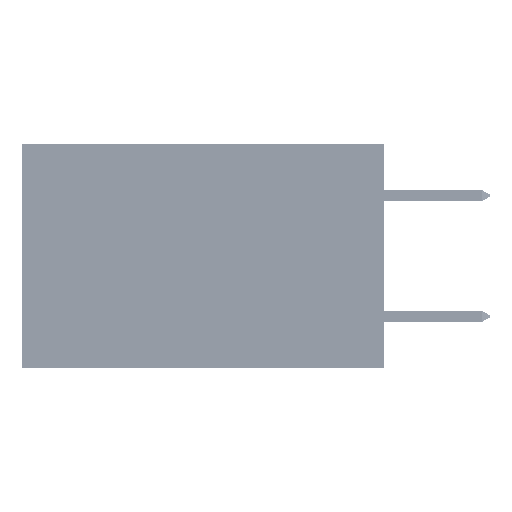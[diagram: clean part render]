
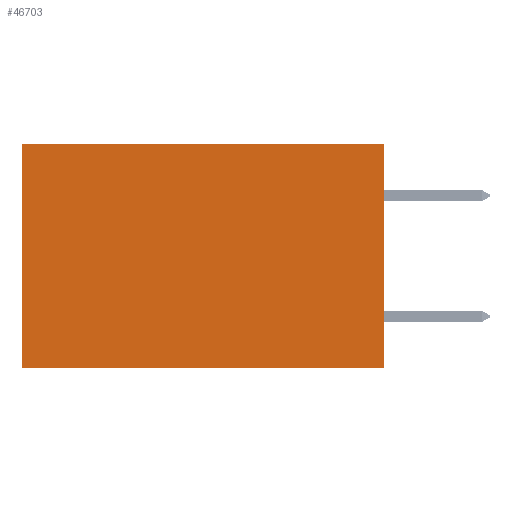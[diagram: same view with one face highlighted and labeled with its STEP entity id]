
A CAD part, left-side view. The second image highlights one B-rep face of the part: STEP entity #46703.
In plain terms, the highlighted planar face has unit normal (-1, 0, 0).
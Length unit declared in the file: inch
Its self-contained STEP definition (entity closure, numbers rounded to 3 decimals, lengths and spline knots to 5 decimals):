
#183 = CARTESIAN_POINT ( 'NONE',  ( 0.2875, 0., 0. ) ) ;
#894 = CARTESIAN_POINT ( 'NONE',  ( 0.2875, 0., -0.37 ) ) ;
#3247 = CARTESIAN_POINT ( 'NONE',  ( 0.2875, 0., 0. ) ) ;
#5212 = EDGE_LOOP ( 'NONE', ( #28532, #8149, #8912, #12407 ) ) ;
#7682 = PLANE ( 'NONE',  #45016 ) ;
#7982 = CARTESIAN_POINT ( 'NONE',  ( 0.2875, 0.6, 0. ) ) ;
#8149 = ORIENTED_EDGE ( 'NONE', *, *, #19596, .F. ) ;
#8912 = ORIENTED_EDGE ( 'NONE', *, *, #36815, .F. ) ;
#11177 = DIRECTION ( 'NONE',  ( 1., 0., 0. ) ) ;
#11255 = EDGE_CURVE ( 'NONE', #34140, #37535, #30874, .T. ) ;
#12407 = ORIENTED_EDGE ( 'NONE', *, *, #11255, .T. ) ;
#12675 = VECTOR ( 'NONE', #35215, 39.37008 ) ;
#12877 = EDGE_CURVE ( 'NONE', #37535, #36492, #42165, .T. ) ;
#14419 = FACE_OUTER_BOUND ( 'NONE', #5212, .T. ) ;
#14825 = VECTOR ( 'NONE', #38874, 39.37008 ) ;
#16137 = VERTEX_POINT ( 'NONE', #894 ) ;
#19596 = EDGE_CURVE ( 'NONE', #16137, #36492, #31246, .T. ) ;
#21498 = DIRECTION ( 'NONE',  ( 0., 1., 0. ) ) ;
#24395 = VECTOR ( 'NONE', #21498, 39.37008 ) ;
#25316 = CARTESIAN_POINT ( 'NONE',  ( 0.2875, 0., -0.37 ) ) ;
#25804 = DIRECTION ( 'NONE',  ( 0., 0., -1. ) ) ;
#28532 = ORIENTED_EDGE ( 'NONE', *, *, #12877, .T. ) ;
#29290 = DIRECTION ( 'NONE',  ( 0., 0., -1. ) ) ;
#30784 = VECTOR ( 'NONE', #25804, 39.37008 ) ;
#30874 = LINE ( 'NONE', #3247, #12675 ) ;
#31246 = LINE ( 'NONE', #25316, #24395 ) ;
#34140 = VERTEX_POINT ( 'NONE', #36413 ) ;
#35215 = DIRECTION ( 'NONE',  ( 0., 1., 0. ) ) ;
#35524 = CARTESIAN_POINT ( 'NONE',  ( 0.2875, 0., 0. ) ) ;
#36413 = CARTESIAN_POINT ( 'NONE',  ( 0.2875, 0., 0. ) ) ;
#36492 = VERTEX_POINT ( 'NONE', #37787 ) ;
#36628 = CARTESIAN_POINT ( 'NONE',  ( 0.2875, 0.6, 0. ) ) ;
#36815 = EDGE_CURVE ( 'NONE', #34140, #16137, #44973, .T. ) ;
#37535 = VERTEX_POINT ( 'NONE', #7982 ) ;
#37787 = CARTESIAN_POINT ( 'NONE',  ( 0.2875, 0.6, -0.37 ) ) ;
#38874 = DIRECTION ( 'NONE',  ( 0., 0., -1. ) ) ;
#42165 = LINE ( 'NONE', #36628, #30784 ) ;
#44973 = LINE ( 'NONE', #35524, #14825 ) ;
#45016 = AXIS2_PLACEMENT_3D ( 'NONE', #183, #11177, #29290 ) ;
#46703 = ADVANCED_FACE ( 'NONE', ( #14419 ), #7682, .F. ) ;
